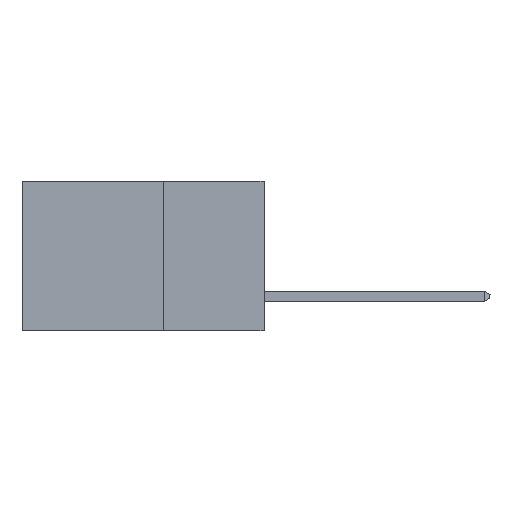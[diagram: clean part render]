
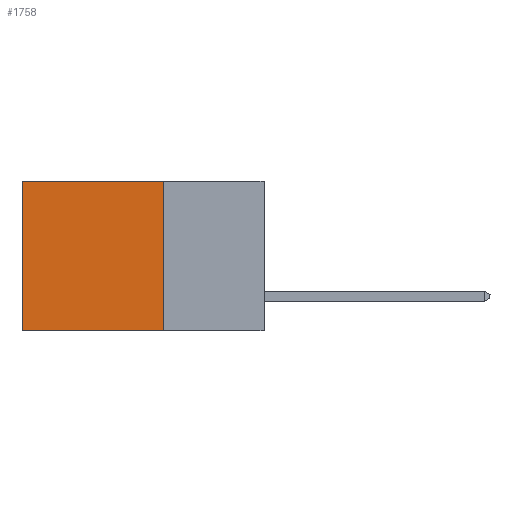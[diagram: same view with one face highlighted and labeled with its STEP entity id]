
A CAD part, left-side view. The second image highlights one B-rep face of the part: STEP entity #1758.
In plain terms, the highlighted planar face has unit normal (-1, 0, 0).
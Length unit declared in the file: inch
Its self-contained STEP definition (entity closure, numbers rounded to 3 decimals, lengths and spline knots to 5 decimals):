
#156 = ORIENTED_EDGE ( 'NONE', *, *, #12475, .F. ) ;
#574 = DIRECTION ( 'NONE',  ( 0., 0., -1. ) ) ;
#704 = LINE ( 'NONE', #3402, #11265 ) ;
#1758 = ADVANCED_FACE ( 'NONE', ( #3058 ), #6922, .F. ) ;
#1804 = DIRECTION ( 'NONE',  ( 0., 0., -1. ) ) ;
#1938 = ORIENTED_EDGE ( 'NONE', *, *, #8582, .T. ) ;
#1999 = CARTESIAN_POINT ( 'NONE',  ( 0.298, 0.6, -0.37 ) ) ;
#2016 = CARTESIAN_POINT ( 'NONE',  ( 0.298, 0.6, 0. ) ) ;
#3058 = FACE_OUTER_BOUND ( 'NONE', #9345, .T. ) ;
#3402 = CARTESIAN_POINT ( 'NONE',  ( 0.298, 0.25, 0. ) ) ;
#3512 = LINE ( 'NONE', #8248, #15783 ) ;
#4764 = EDGE_CURVE ( 'NONE', #9480, #15257, #704, .T. ) ;
#5243 = VECTOR ( 'NONE', #11870, 39.37008 ) ;
#6922 = PLANE ( 'NONE',  #10054 ) ;
#8248 = CARTESIAN_POINT ( 'NONE',  ( 0.298, 0.25, 0. ) ) ;
#8582 = EDGE_CURVE ( 'NONE', #15257, #12750, #11966, .T. ) ;
#8837 = VECTOR ( 'NONE', #14286, 39.37008 ) ;
#8953 = EDGE_CURVE ( 'NONE', #15325, #12750, #15140, .T. ) ;
#9345 = EDGE_LOOP ( 'NONE', ( #1938, #12730, #156, #16138 ) ) ;
#9480 = VERTEX_POINT ( 'NONE', #13480 ) ;
#10054 = AXIS2_PLACEMENT_3D ( 'NONE', #15714, #14470, #1804 ) ;
#11265 = VECTOR ( 'NONE', #12274, 39.37008 ) ;
#11815 = CARTESIAN_POINT ( 'NONE',  ( 0.298, 0.6, 0. ) ) ;
#11870 = DIRECTION ( 'NONE',  ( 0., 0., -1. ) ) ;
#11966 = LINE ( 'NONE', #11815, #5243 ) ;
#12274 = DIRECTION ( 'NONE',  ( 0., 1., 0. ) ) ;
#12475 = EDGE_CURVE ( 'NONE', #9480, #15325, #3512, .T. ) ;
#12730 = ORIENTED_EDGE ( 'NONE', *, *, #8953, .F. ) ;
#12750 = VERTEX_POINT ( 'NONE', #1999 ) ;
#13480 = CARTESIAN_POINT ( 'NONE',  ( 0.298, 0.25, 0. ) ) ;
#14286 = DIRECTION ( 'NONE',  ( 0., 1., 0. ) ) ;
#14470 = DIRECTION ( 'NONE',  ( 1., 0., 0. ) ) ;
#14989 = CARTESIAN_POINT ( 'NONE',  ( 0.298, 0.25, -0.37 ) ) ;
#14995 = CARTESIAN_POINT ( 'NONE',  ( 0.298, 0.25, -0.37 ) ) ;
#15140 = LINE ( 'NONE', #14989, #8837 ) ;
#15257 = VERTEX_POINT ( 'NONE', #2016 ) ;
#15325 = VERTEX_POINT ( 'NONE', #14995 ) ;
#15714 = CARTESIAN_POINT ( 'NONE',  ( 0.298, 0.25, 0. ) ) ;
#15783 = VECTOR ( 'NONE', #574, 39.37008 ) ;
#16138 = ORIENTED_EDGE ( 'NONE', *, *, #4764, .T. ) ;
